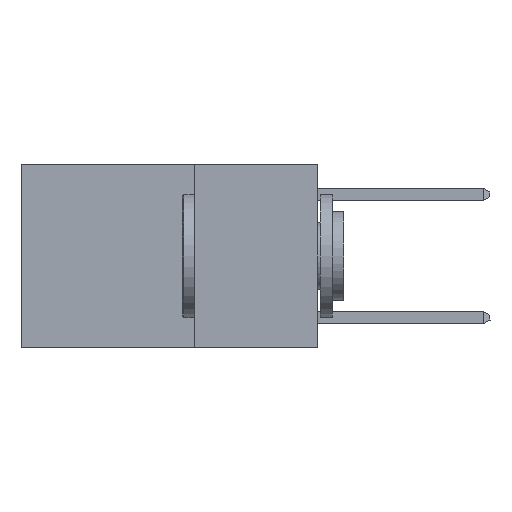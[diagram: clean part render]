
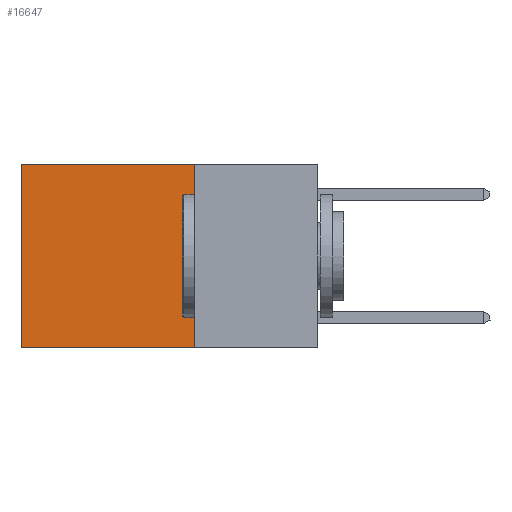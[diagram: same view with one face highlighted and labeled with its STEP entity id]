
A CAD part, left-side view. The second image highlights one B-rep face of the part: STEP entity #16647.
In plain terms, the highlighted planar face has unit normal (-1, 0, 0).
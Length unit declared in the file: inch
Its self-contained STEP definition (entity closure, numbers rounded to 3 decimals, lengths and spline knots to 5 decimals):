
#651 = ORIENTED_EDGE ( 'NONE', *, *, #22135, .T. ) ;
#780 = VERTEX_POINT ( 'NONE', #23184 ) ;
#824 = ORIENTED_EDGE ( 'NONE', *, *, #23014, .F. ) ;
#1451 = CARTESIAN_POINT ( 'NONE',  ( 0.2625, 0.6, -0.37 ) ) ;
#2692 = VERTEX_POINT ( 'NONE', #1451 ) ;
#2988 = CARTESIAN_POINT ( 'NONE',  ( 0.2625, 0.25, 0. ) ) ;
#3438 = VERTEX_POINT ( 'NONE', #5705 ) ;
#3747 = VECTOR ( 'NONE', #14025, 39.37008 ) ;
#4663 = DIRECTION ( 'NONE',  ( 0., 1., 0. ) ) ;
#5636 = CARTESIAN_POINT ( 'NONE',  ( 0.2625, 0.6, 0. ) ) ;
#5705 = CARTESIAN_POINT ( 'NONE',  ( 0.2625, 0.25, 0. ) ) ;
#6373 = FACE_OUTER_BOUND ( 'NONE', #13131, .T. ) ;
#6808 = ORIENTED_EDGE ( 'NONE', *, *, #15596, .F. ) ;
#7266 = DIRECTION ( 'NONE',  ( 0., 0., -1. ) ) ;
#7513 = CARTESIAN_POINT ( 'NONE',  ( 0.2625, 0.6, 0. ) ) ;
#7578 = LINE ( 'NONE', #2988, #17535 ) ;
#8682 = PLANE ( 'NONE',  #16772 ) ;
#10600 = VECTOR ( 'NONE', #4663, 39.37008 ) ;
#10725 = DIRECTION ( 'NONE',  ( 0., 0., -1. ) ) ;
#11227 = VERTEX_POINT ( 'NONE', #5636 ) ;
#11966 = CARTESIAN_POINT ( 'NONE',  ( 0.2625, 0.25, -0.37 ) ) ;
#12676 = CARTESIAN_POINT ( 'NONE',  ( 0.2625, 0.25, 0. ) ) ;
#13131 = EDGE_LOOP ( 'NONE', ( #18998, #824, #6808, #651 ) ) ;
#14025 = DIRECTION ( 'NONE',  ( 0., 1., 0. ) ) ;
#14885 = LINE ( 'NONE', #7513, #19313 ) ;
#15596 = EDGE_CURVE ( 'NONE', #3438, #780, #7578, .T. ) ;
#16647 = ADVANCED_FACE ( 'NONE', ( #6373 ), #8682, .F. ) ;
#16723 = CARTESIAN_POINT ( 'NONE',  ( 0.2625, 0.25, 0. ) ) ;
#16772 = AXIS2_PLACEMENT_3D ( 'NONE', #12676, #22305, #10725 ) ;
#17535 = VECTOR ( 'NONE', #7266, 39.37008 ) ;
#17910 = EDGE_CURVE ( 'NONE', #11227, #2692, #14885, .T. ) ;
#18998 = ORIENTED_EDGE ( 'NONE', *, *, #17910, .T. ) ;
#19313 = VECTOR ( 'NONE', #21255, 39.37008 ) ;
#21255 = DIRECTION ( 'NONE',  ( 0., 0., -1. ) ) ;
#22135 = EDGE_CURVE ( 'NONE', #3438, #11227, #25147, .T. ) ;
#22305 = DIRECTION ( 'NONE',  ( 1., 0., 0. ) ) ;
#23014 = EDGE_CURVE ( 'NONE', #780, #2692, #24554, .T. ) ;
#23184 = CARTESIAN_POINT ( 'NONE',  ( 0.2625, 0.25, -0.37 ) ) ;
#24554 = LINE ( 'NONE', #11966, #3747 ) ;
#25147 = LINE ( 'NONE', #16723, #10600 ) ;
